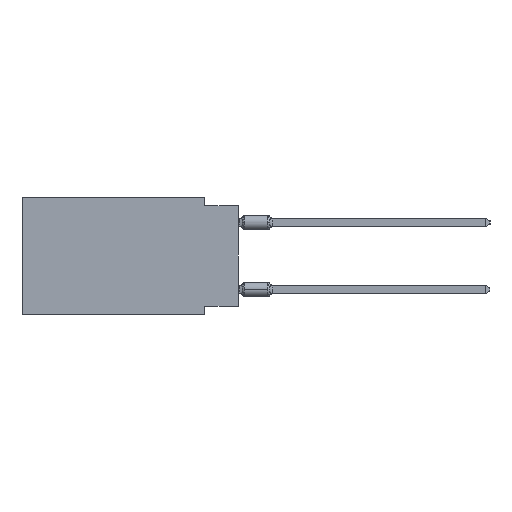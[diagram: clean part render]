
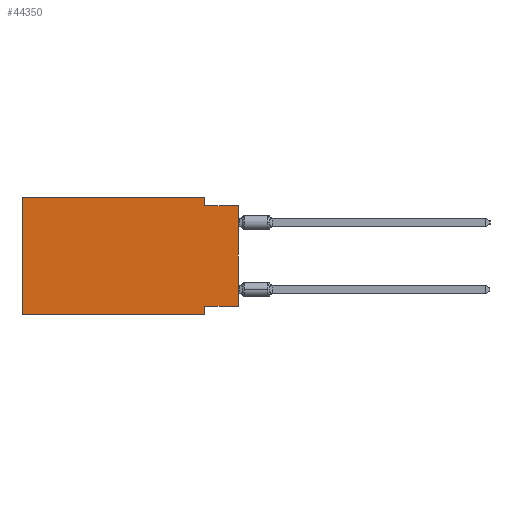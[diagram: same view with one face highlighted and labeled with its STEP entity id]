
A CAD part, left-side view. The second image highlights one B-rep face of the part: STEP entity #44350.
In plain terms, the highlighted planar face has unit normal (-1, 0, 0).
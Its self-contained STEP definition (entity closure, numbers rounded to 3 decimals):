
#174 = VERTEX_POINT ( 'NONE', #62973 ) ;
#290 = DIRECTION ( 'NONE',  ( 0., -1., 0. ) ) ;
#1598 = CARTESIAN_POINT ( 'NONE',  ( 0., 0., -0.635 ) ) ;
#2342 = DIRECTION ( 'NONE',  ( 0., 1., 0. ) ) ;
#5784 = VERTEX_POINT ( 'NONE', #62883 ) ;
#5861 = LINE ( 'NONE', #51748, #9309 ) ;
#6146 = VECTOR ( 'NONE', #16583, 1000. ) ;
#7657 = VECTOR ( 'NONE', #39314, 1000. ) ;
#9309 = VECTOR ( 'NONE', #18043, 1000. ) ;
#11265 = LINE ( 'NONE', #1598, #55396 ) ;
#11595 = CARTESIAN_POINT ( 'NONE',  ( 0., 16.383, 0. ) ) ;
#11827 = ORIENTED_EDGE ( 'NONE', *, *, #56222, .F. ) ;
#11973 = CARTESIAN_POINT ( 'NONE',  ( 0., 16.383, 0. ) ) ;
#13886 = VECTOR ( 'NONE', #49234, 1000. ) ;
#16583 = DIRECTION ( 'NONE',  ( 0., -1., 0. ) ) ;
#18003 = LINE ( 'NONE', #53263, #13886 ) ;
#18043 = DIRECTION ( 'NONE',  ( 0., 0., 1. ) ) ;
#18950 = CARTESIAN_POINT ( 'NONE',  ( 0., 2.54, -0.635 ) ) ;
#22477 = EDGE_CURVE ( 'NONE', #38267, #5784, #47267, .T. ) ;
#23363 = LINE ( 'NONE', #24007, #7657 ) ;
#23919 = EDGE_CURVE ( 'NONE', #174, #5784, #23363, .T. ) ;
#24007 = CARTESIAN_POINT ( 'NONE',  ( 0., 16.383, -8.89 ) ) ;
#26134 = CARTESIAN_POINT ( 'NONE',  ( 0., 2.54, 0. ) ) ;
#26646 = LINE ( 'NONE', #58224, #63430 ) ;
#28624 = CARTESIAN_POINT ( 'NONE',  ( 0., 2.54, -8.255 ) ) ;
#29356 = ORIENTED_EDGE ( 'NONE', *, *, #35164, .T. ) ;
#30849 = DIRECTION ( 'NONE',  ( 0., 0., 1. ) ) ;
#31985 = EDGE_LOOP ( 'NONE', ( #29356, #32312, #48802, #33423, #42322, #57728, #42206, #11827 ) ) ;
#32073 = CARTESIAN_POINT ( 'NONE',  ( 0., 0., -0.635 ) ) ;
#32238 = DIRECTION ( 'NONE',  ( 1., 0., 0. ) ) ;
#32312 = ORIENTED_EDGE ( 'NONE', *, *, #33298, .F. ) ;
#32555 = VECTOR ( 'NONE', #30849, 1000. ) ;
#33108 = VERTEX_POINT ( 'NONE', #18950 ) ;
#33298 = EDGE_CURVE ( 'NONE', #33108, #47028, #11265, .T. ) ;
#33423 = ORIENTED_EDGE ( 'NONE', *, *, #49800, .F. ) ;
#33657 = VERTEX_POINT ( 'NONE', #26134 ) ;
#35164 = EDGE_CURVE ( 'NONE', #45878, #47028, #61112, .T. ) ;
#36193 = VECTOR ( 'NONE', #37605, 1000. ) ;
#37605 = DIRECTION ( 'NONE',  ( 0., 0., -1. ) ) ;
#37827 = CARTESIAN_POINT ( 'NONE',  ( 0., 16.383, 0. ) ) ;
#38267 = VERTEX_POINT ( 'NONE', #28624 ) ;
#38445 = AXIS2_PLACEMENT_3D ( 'NONE', #11973, #32238, #47534 ) ;
#39314 = DIRECTION ( 'NONE',  ( 0., -1., 0. ) ) ;
#42171 = LINE ( 'NONE', #11595, #6146 ) ;
#42206 = ORIENTED_EDGE ( 'NONE', *, *, #22477, .F. ) ;
#42322 = ORIENTED_EDGE ( 'NONE', *, *, #50155, .F. ) ;
#42612 = CARTESIAN_POINT ( 'NONE',  ( 0., 2.54, -8.89 ) ) ;
#44350 = ADVANCED_FACE ( 'NONE', ( #57544 ), #62851, .F. ) ;
#45878 = VERTEX_POINT ( 'NONE', #52175 ) ;
#47028 = VERTEX_POINT ( 'NONE', #32073 ) ;
#47267 = LINE ( 'NONE', #42612, #36193 ) ;
#47485 = EDGE_CURVE ( 'NONE', #33657, #33108, #18003, .T. ) ;
#47534 = DIRECTION ( 'NONE',  ( 0., 0., -1. ) ) ;
#48802 = ORIENTED_EDGE ( 'NONE', *, *, #47485, .F. ) ;
#49234 = DIRECTION ( 'NONE',  ( 0., 0., -1. ) ) ;
#49800 = EDGE_CURVE ( 'NONE', #64073, #33657, #42171, .T. ) ;
#50155 = EDGE_CURVE ( 'NONE', #174, #64073, #5861, .T. ) ;
#51748 = CARTESIAN_POINT ( 'NONE',  ( 0., 16.383, 0. ) ) ;
#52175 = CARTESIAN_POINT ( 'NONE',  ( 0., 0., -8.255 ) ) ;
#53263 = CARTESIAN_POINT ( 'NONE',  ( 0., 2.54, 0. ) ) ;
#55396 = VECTOR ( 'NONE', #290, 1000. ) ;
#56131 = CARTESIAN_POINT ( 'NONE',  ( 0., 0., 0. ) ) ;
#56222 = EDGE_CURVE ( 'NONE', #45878, #38267, #26646, .T. ) ;
#57544 = FACE_OUTER_BOUND ( 'NONE', #31985, .T. ) ;
#57728 = ORIENTED_EDGE ( 'NONE', *, *, #23919, .T. ) ;
#58224 = CARTESIAN_POINT ( 'NONE',  ( 0., 0., -8.255 ) ) ;
#61112 = LINE ( 'NONE', #56131, #32555 ) ;
#62851 = PLANE ( 'NONE',  #38445 ) ;
#62883 = CARTESIAN_POINT ( 'NONE',  ( 0., 2.54, -8.89 ) ) ;
#62973 = CARTESIAN_POINT ( 'NONE',  ( 0., 16.383, -8.89 ) ) ;
#63430 = VECTOR ( 'NONE', #2342, 1000. ) ;
#64073 = VERTEX_POINT ( 'NONE', #37827 ) ;
